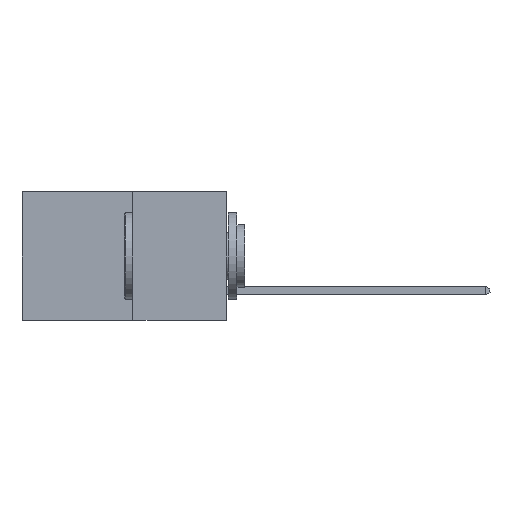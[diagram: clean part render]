
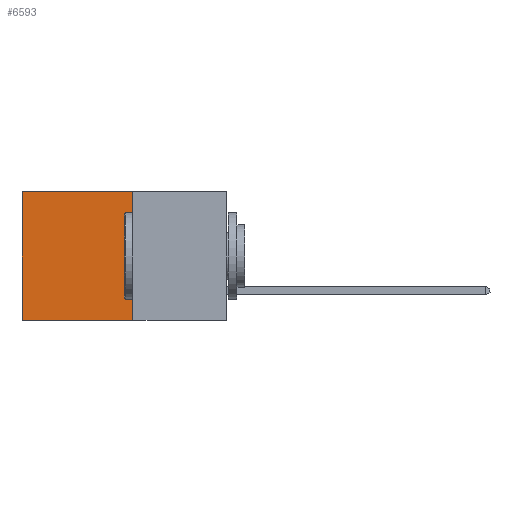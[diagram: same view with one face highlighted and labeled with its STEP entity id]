
A CAD part, left-side view. The second image highlights one B-rep face of the part: STEP entity #6593.
In plain terms, the highlighted planar face has unit normal (-1, 0, 0).
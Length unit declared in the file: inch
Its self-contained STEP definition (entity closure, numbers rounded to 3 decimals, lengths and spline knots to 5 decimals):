
#198 = ORIENTED_EDGE ( 'NONE', *, *, #3419, .F. ) ;
#549 = DIRECTION ( 'NONE',  ( 0., 0., -1. ) ) ;
#565 = DIRECTION ( 'NONE',  ( 1., 0., 0. ) ) ;
#611 = CARTESIAN_POINT ( 'NONE',  ( 0.277, 0.27, -0.37 ) ) ;
#682 = PLANE ( 'NONE',  #12014 ) ;
#951 = VERTEX_POINT ( 'NONE', #4380 ) ;
#2104 = CARTESIAN_POINT ( 'NONE',  ( 0.277, 0.27, -0.37 ) ) ;
#2377 = ORIENTED_EDGE ( 'NONE', *, *, #11483, .T. ) ;
#2746 = DIRECTION ( 'NONE',  ( 0., 1., 0. ) ) ;
#2773 = CARTESIAN_POINT ( 'NONE',  ( 0.277, 0.27, 0. ) ) ;
#3057 = LINE ( 'NONE', #2773, #5295 ) ;
#3419 = EDGE_CURVE ( 'NONE', #5370, #8927, #4185, .T. ) ;
#3430 = CARTESIAN_POINT ( 'NONE',  ( 0.277, 0.27, -0.37 ) ) ;
#3946 = FACE_OUTER_BOUND ( 'NONE', #4769, .T. ) ;
#4185 = LINE ( 'NONE', #2104, #8891 ) ;
#4380 = CARTESIAN_POINT ( 'NONE',  ( 0.277, 0.59, 0. ) ) ;
#4414 = DIRECTION ( 'NONE',  ( 0., 1., 0. ) ) ;
#4769 = EDGE_LOOP ( 'NONE', ( #2377, #4926, #198, #10194 ) ) ;
#4926 = ORIENTED_EDGE ( 'NONE', *, *, #8747, .F. ) ;
#5295 = VECTOR ( 'NONE', #2746, 39.37008 ) ;
#5370 = VERTEX_POINT ( 'NONE', #8685 ) ;
#5689 = CARTESIAN_POINT ( 'NONE',  ( 0.277, 0.27, -0.37 ) ) ;
#5955 = LINE ( 'NONE', #3430, #10609 ) ;
#6277 = EDGE_CURVE ( 'NONE', #5370, #951, #3057, .T. ) ;
#6593 = ADVANCED_FACE ( 'NONE', ( #3946 ), #682, .F. ) ;
#7380 = CARTESIAN_POINT ( 'NONE',  ( 0.277, 0.59, -0.37 ) ) ;
#7524 = CARTESIAN_POINT ( 'NONE',  ( 0.277, 0.59, -0.37 ) ) ;
#7922 = VECTOR ( 'NONE', #8487, 39.37008 ) ;
#8165 = VERTEX_POINT ( 'NONE', #7380 ) ;
#8487 = DIRECTION ( 'NONE',  ( 0., 0., -1. ) ) ;
#8685 = CARTESIAN_POINT ( 'NONE',  ( 0.277, 0.27, 0. ) ) ;
#8747 = EDGE_CURVE ( 'NONE', #8927, #8165, #5955, .T. ) ;
#8891 = VECTOR ( 'NONE', #11785, 39.37008 ) ;
#8927 = VERTEX_POINT ( 'NONE', #5689 ) ;
#10194 = ORIENTED_EDGE ( 'NONE', *, *, #6277, .T. ) ;
#10387 = LINE ( 'NONE', #7524, #7922 ) ;
#10609 = VECTOR ( 'NONE', #4414, 39.37008 ) ;
#11483 = EDGE_CURVE ( 'NONE', #951, #8165, #10387, .T. ) ;
#11785 = DIRECTION ( 'NONE',  ( 0., 0., -1. ) ) ;
#12014 = AXIS2_PLACEMENT_3D ( 'NONE', #611, #565, #549 ) ;
